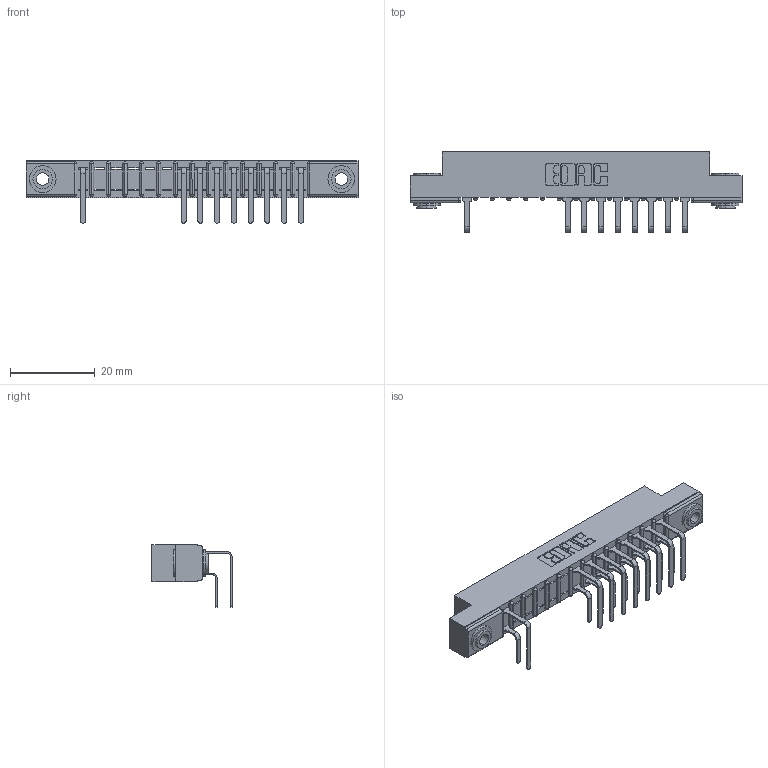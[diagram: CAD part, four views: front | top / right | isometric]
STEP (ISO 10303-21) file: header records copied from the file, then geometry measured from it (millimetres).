
FILE_DESCRIPTION (( 'STEP AP203' ), '1' );
FILE_NAME ('357-014-558-103.STEP', '2018-08-07T23:37:26', ( '' ), ( '' ), 'SwSTEP 2.0', 'SolidWorks 2016', '' );
FILE_SCHEMA (( 'CONFIG_CONTROL_DESIGN' ));
Length unit declared in the file: inch
Products named in the file (5): 307-290-001_558 - 2 (Single); 345-250-002_345-250-002-102; 357-014-558-103; 307 Part_.156 Dia Mounting Holes; 307-290-001_558 559 - 1 (Single)
Assembly tree (21 placements, depth 2):
  357-014-558-103
    307 Part_.156 Dia Mounting Holes
    307-290-001_558 559 - 1 (Single)  x9
    307-290-001_558 - 2 (Single)  x9
    345-250-002_345-250-002-102  x2
Bounding box: 78.49 x 18.96 x 14.81 mm (x, y, z)
Volume: 5086.3 mm3; surface area: 8498.4 mm2
Topology: 21 solids, 21 shells, 1185 faces, 3311 edges, 2138 vertices
Faces by surface type: plane 748, cylinder 399, sphere 30, cone 8
Entity records: 18094 total; most frequent: CARTESIAN_POINT 2995, ORIENTED_EDGE 2966, DIRECTION 2949, EDGE_CURVE 1483, LINE 1117, VECTOR 1117, VERTEX_POINT 962, AXIS2_PLACEMENT_3D 916
